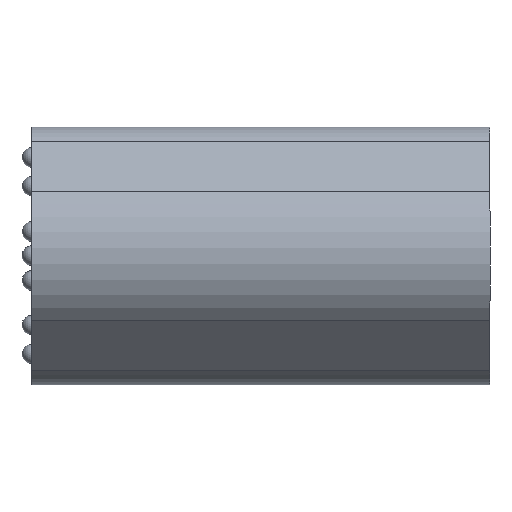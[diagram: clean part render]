
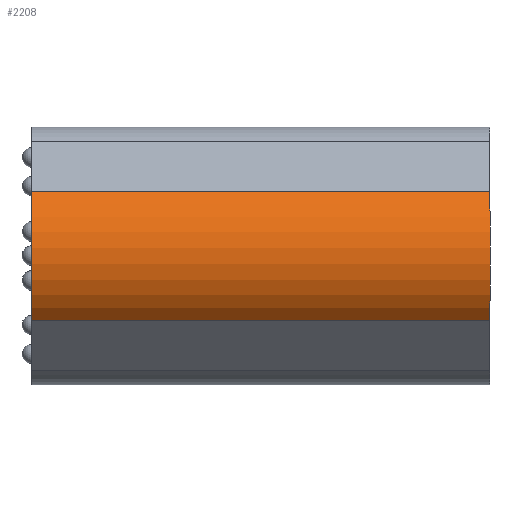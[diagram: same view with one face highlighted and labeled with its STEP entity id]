
A CAD part, left-side view. The second image highlights one B-rep face of the part: STEP entity #2208.
In plain terms, the highlighted cylindrical face has radius 18.575 mm (diameter 37.15 mm), a partial arc.
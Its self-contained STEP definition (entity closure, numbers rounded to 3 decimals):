
#19 = DIRECTION ( 'NONE',  ( 0., -1., 0. ) ) ;
#27 = DIRECTION ( 'NONE',  ( 0., -1., 0. ) ) ;
#145 = LINE ( 'NONE', #1143, #1636 ) ;
#188 = EDGE_LOOP ( 'NONE', ( #236, #247, #265, #499 ) ) ;
#218 = DIRECTION ( 'NONE',  ( 0., -1., 0. ) ) ;
#236 = ORIENTED_EDGE ( 'NONE', *, *, #2167, .T. ) ;
#247 = ORIENTED_EDGE ( 'NONE', *, *, #1079, .T. ) ;
#260 = CARTESIAN_POINT ( 'NONE',  ( -193.405, -18.876, 4.547 ) ) ;
#265 = ORIENTED_EDGE ( 'NONE', *, *, #936, .F. ) ;
#368 = VERTEX_POINT ( 'NONE', #788 ) ;
#370 = CYLINDRICAL_SURFACE ( 'NONE', #798, 18.575 ) ;
#391 = DIRECTION ( 'NONE',  ( 0., 0., 1. ) ) ;
#427 = DIRECTION ( 'NONE',  ( 0., 0., 1. ) ) ;
#499 = ORIENTED_EDGE ( 'NONE', *, *, #1243, .F. ) ;
#788 = CARTESIAN_POINT ( 'NONE',  ( -206.54, -18.876, 17.682 ) ) ;
#798 = AXIS2_PLACEMENT_3D ( 'NONE', #1728, #27, #391 ) ;
#836 = VERTEX_POINT ( 'NONE', #1873 ) ;
#936 = EDGE_CURVE ( 'NONE', #1862, #368, #145, .T. ) ;
#955 = VERTEX_POINT ( 'NONE', #1156 ) ;
#989 = VECTOR ( 'NONE', #19, 1000. ) ;
#993 = CIRCLE ( 'NONE', #1640, 18.575 ) ;
#1046 = DIRECTION ( 'NONE',  ( 0., 1., 0. ) ) ;
#1079 = EDGE_CURVE ( 'NONE', #955, #368, #1343, .T. ) ;
#1143 = CARTESIAN_POINT ( 'NONE',  ( -206.54, -231.033, 17.682 ) ) ;
#1156 = CARTESIAN_POINT ( 'NONE',  ( -206.54, -18.876, -8.587 ) ) ;
#1243 = EDGE_CURVE ( 'NONE', #836, #1862, #993, .T. ) ;
#1330 = CARTESIAN_POINT ( 'NONE',  ( -206.54, 74.373, 17.682 ) ) ;
#1343 = CIRCLE ( 'NONE', #1722, 18.575 ) ;
#1492 = CARTESIAN_POINT ( 'NONE',  ( -206.54, 153.844, -8.587 ) ) ;
#1500 = LINE ( 'NONE', #1492, #989 ) ;
#1567 = DIRECTION ( 'NONE',  ( 0., 1., 0. ) ) ;
#1636 = VECTOR ( 'NONE', #218, 1000. ) ;
#1640 = AXIS2_PLACEMENT_3D ( 'NONE', #2207, #1046, #2370 ) ;
#1722 = AXIS2_PLACEMENT_3D ( 'NONE', #260, #1567, #427 ) ;
#1728 = CARTESIAN_POINT ( 'NONE',  ( -193.405, 153.844, 4.547 ) ) ;
#1862 = VERTEX_POINT ( 'NONE', #1330 ) ;
#1873 = CARTESIAN_POINT ( 'NONE',  ( -206.54, 74.373, -8.587 ) ) ;
#1907 = FACE_OUTER_BOUND ( 'NONE', #188, .T. ) ;
#2167 = EDGE_CURVE ( 'NONE', #836, #955, #1500, .T. ) ;
#2207 = CARTESIAN_POINT ( 'NONE',  ( -193.405, 74.373, 4.547 ) ) ;
#2208 = ADVANCED_FACE ( 'NONE', ( #1907 ), #370, .T. ) ;
#2370 = DIRECTION ( 'NONE',  ( 0., 0., 1. ) ) ;
